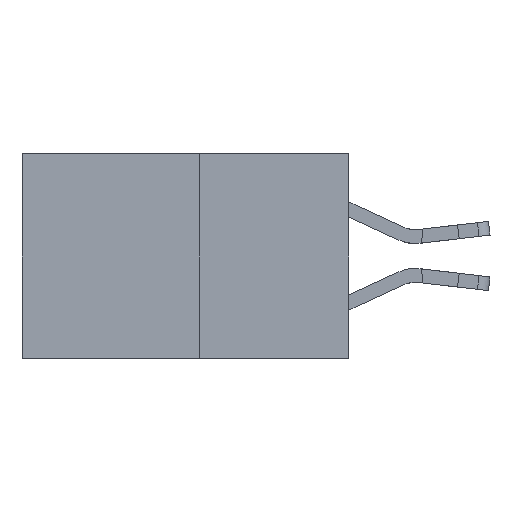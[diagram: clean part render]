
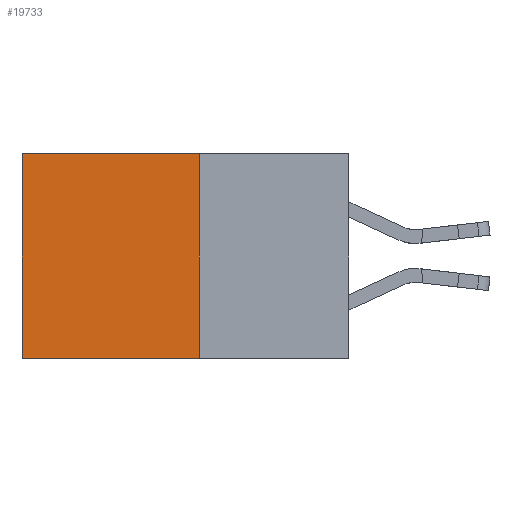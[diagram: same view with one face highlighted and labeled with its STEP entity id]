
A CAD part, left-side view. The second image highlights one B-rep face of the part: STEP entity #19733.
In plain terms, the highlighted planar face has unit normal (-1, 0, 0).
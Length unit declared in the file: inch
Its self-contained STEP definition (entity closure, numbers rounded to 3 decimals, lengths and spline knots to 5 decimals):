
#815 = VERTEX_POINT ( 'NONE', #14693 ) ;
#1055 = CARTESIAN_POINT ( 'NONE',  ( 0.277, 0.27, -0.37 ) ) ;
#1151 = PLANE ( 'NONE',  #11570 ) ;
#1343 = ORIENTED_EDGE ( 'NONE', *, *, #4198, .T. ) ;
#1579 = ORIENTED_EDGE ( 'NONE', *, *, #5556, .F. ) ;
#2393 = ORIENTED_EDGE ( 'NONE', *, *, #6253, .F. ) ;
#2737 = ORIENTED_EDGE ( 'NONE', *, *, #22540, .T. ) ;
#2985 = DIRECTION ( 'NONE',  ( 0., 1., 0. ) ) ;
#3952 = LINE ( 'NONE', #5831, #22358 ) ;
#4198 = EDGE_CURVE ( 'NONE', #17866, #12076, #3952, .T. ) ;
#5420 = FACE_OUTER_BOUND ( 'NONE', #13367, .T. ) ;
#5556 = EDGE_CURVE ( 'NONE', #15720, #12076, #19298, .T. ) ;
#5831 = CARTESIAN_POINT ( 'NONE',  ( 0.277, 0.59, -0.37 ) ) ;
#6253 = EDGE_CURVE ( 'NONE', #815, #15720, #18998, .T. ) ;
#7904 = DIRECTION ( 'NONE',  ( 0., 0., -1. ) ) ;
#8525 = CARTESIAN_POINT ( 'NONE',  ( 0.277, 0.27, -0.37 ) ) ;
#10366 = DIRECTION ( 'NONE',  ( 0., 0., -1. ) ) ;
#10525 = VECTOR ( 'NONE', #2985, 39.37008 ) ;
#10847 = CARTESIAN_POINT ( 'NONE',  ( 0.277, 0.59, 0. ) ) ;
#11570 = AXIS2_PLACEMENT_3D ( 'NONE', #8525, #20872, #10366 ) ;
#12076 = VERTEX_POINT ( 'NONE', #17004 ) ;
#13367 = EDGE_LOOP ( 'NONE', ( #1343, #1579, #2393, #2737 ) ) ;
#13424 = CARTESIAN_POINT ( 'NONE',  ( 0.277, 0.27, -0.37 ) ) ;
#13624 = LINE ( 'NONE', #19642, #14155 ) ;
#14155 = VECTOR ( 'NONE', #17863, 39.37008 ) ;
#14323 = VECTOR ( 'NONE', #21711, 39.37008 ) ;
#14693 = CARTESIAN_POINT ( 'NONE',  ( 0.277, 0.27, 0. ) ) ;
#15720 = VERTEX_POINT ( 'NONE', #1055 ) ;
#17004 = CARTESIAN_POINT ( 'NONE',  ( 0.277, 0.59, -0.37 ) ) ;
#17863 = DIRECTION ( 'NONE',  ( 0., 1., 0. ) ) ;
#17866 = VERTEX_POINT ( 'NONE', #10847 ) ;
#18998 = LINE ( 'NONE', #19101, #14323 ) ;
#19101 = CARTESIAN_POINT ( 'NONE',  ( 0.277, 0.27, -0.37 ) ) ;
#19298 = LINE ( 'NONE', #13424, #10525 ) ;
#19642 = CARTESIAN_POINT ( 'NONE',  ( 0.277, 0.27, 0. ) ) ;
#19733 = ADVANCED_FACE ( 'NONE', ( #5420 ), #1151, .F. ) ;
#20872 = DIRECTION ( 'NONE',  ( 1., 0., 0. ) ) ;
#21711 = DIRECTION ( 'NONE',  ( 0., 0., -1. ) ) ;
#22358 = VECTOR ( 'NONE', #7904, 39.37008 ) ;
#22540 = EDGE_CURVE ( 'NONE', #815, #17866, #13624, .T. ) ;
